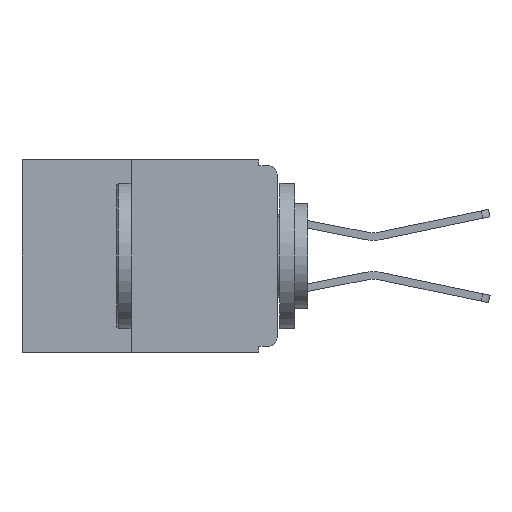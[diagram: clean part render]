
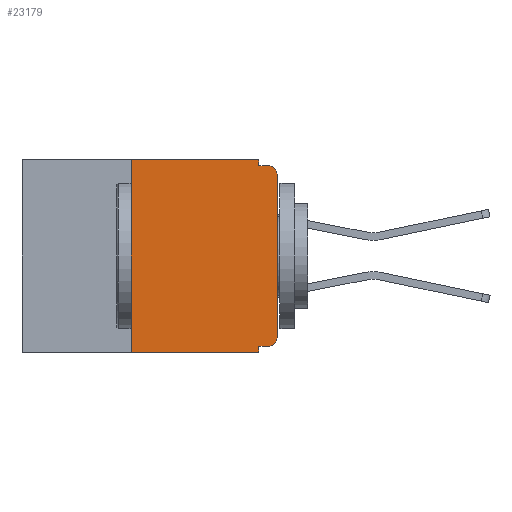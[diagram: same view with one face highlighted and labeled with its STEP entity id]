
A CAD part, left-side view. The second image highlights one B-rep face of the part: STEP entity #23179.
In plain terms, the highlighted planar face has unit normal (-1, 0, 0).
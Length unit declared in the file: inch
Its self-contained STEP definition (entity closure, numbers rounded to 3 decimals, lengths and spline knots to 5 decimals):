
#619 = AXIS2_PLACEMENT_3D ( 'NONE', #27748, #3390, #27098 ) ;
#1403 = ORIENTED_EDGE ( 'NONE', *, *, #21141, .F. ) ;
#2416 = EDGE_CURVE ( 'NONE', #32948, #7726, #2552, .T. ) ;
#2425 = EDGE_CURVE ( 'NONE', #13186, #30338, #24092, .T. ) ;
#2552 = CIRCLE ( 'NONE', #619, 0.015 ) ;
#2761 = LINE ( 'NONE', #4427, #23470 ) ;
#3285 = DIRECTION ( 'NONE',  ( -1., 0., 0. ) ) ;
#3390 = DIRECTION ( 'NONE',  ( -1., 0., 0. ) ) ;
#3770 = LINE ( 'NONE', #6785, #4599 ) ;
#3822 = VERTEX_POINT ( 'NONE', #17124 ) ;
#4195 = CARTESIAN_POINT ( 'NONE',  ( 0., 0.25, -0.33 ) ) ;
#4427 = CARTESIAN_POINT ( 'NONE',  ( 0., 0., -0.32 ) ) ;
#4599 = VECTOR ( 'NONE', #7134, 39.37008 ) ;
#4861 = DIRECTION ( 'NONE',  ( 0., 1., 0. ) ) ;
#5353 = VERTEX_POINT ( 'NONE', #21780 ) ;
#5910 = DIRECTION ( 'NONE',  ( 0., 0., 1. ) ) ;
#5989 = EDGE_CURVE ( 'NONE', #21607, #5353, #2761, .T. ) ;
#6082 = ORIENTED_EDGE ( 'NONE', *, *, #9510, .F. ) ;
#6320 = VECTOR ( 'NONE', #32234, 39.37008 ) ;
#6785 = CARTESIAN_POINT ( 'NONE',  ( 0., 0.031, 0. ) ) ;
#7110 = LINE ( 'NONE', #31302, #33940 ) ;
#7134 = DIRECTION ( 'NONE',  ( 0., 0., -1. ) ) ;
#7726 = VERTEX_POINT ( 'NONE', #27463 ) ;
#8636 = ORIENTED_EDGE ( 'NONE', *, *, #26899, .T. ) ;
#9510 = EDGE_CURVE ( 'NONE', #30338, #3822, #3770, .T. ) ;
#10314 = ORIENTED_EDGE ( 'NONE', *, *, #25846, .F. ) ;
#10710 = ORIENTED_EDGE ( 'NONE', *, *, #17851, .T. ) ;
#11234 = PLANE ( 'NONE',  #32733 ) ;
#13186 = VERTEX_POINT ( 'NONE', #15292 ) ;
#13444 = FACE_OUTER_BOUND ( 'NONE', #34259, .T. ) ;
#13531 = CARTESIAN_POINT ( 'NONE',  ( 0., 0.031, -0.33 ) ) ;
#15292 = CARTESIAN_POINT ( 'NONE',  ( 0., 0.25, 0. ) ) ;
#15488 = CARTESIAN_POINT ( 'NONE',  ( 0., 0.437, -0.33 ) ) ;
#15538 = CIRCLE ( 'NONE', #16472, 0.015 ) ;
#16472 = AXIS2_PLACEMENT_3D ( 'NONE', #19548, #3285, #22234 ) ;
#16754 = DIRECTION ( 'NONE',  ( 0., 0., -1. ) ) ;
#16958 = LINE ( 'NONE', #4195, #23244 ) ;
#17124 = CARTESIAN_POINT ( 'NONE',  ( 0., 0.031, -0.01 ) ) ;
#17563 = ORIENTED_EDGE ( 'NONE', *, *, #5989, .F. ) ;
#17851 = EDGE_CURVE ( 'NONE', #26490, #32948, #23380, .T. ) ;
#17964 = ORIENTED_EDGE ( 'NONE', *, *, #2416, .T. ) ;
#19274 = ORIENTED_EDGE ( 'NONE', *, *, #23769, .T. ) ;
#19548 = CARTESIAN_POINT ( 'NONE',  ( 0., 0.015, -0.305 ) ) ;
#20734 = LINE ( 'NONE', #13531, #6320 ) ;
#21141 = EDGE_CURVE ( 'NONE', #31419, #13186, #16958, .T. ) ;
#21607 = VERTEX_POINT ( 'NONE', #26167 ) ;
#21777 = CARTESIAN_POINT ( 'NONE',  ( 0., 0., -0.305 ) ) ;
#21780 = CARTESIAN_POINT ( 'NONE',  ( 0., 0.031, -0.32 ) ) ;
#22234 = DIRECTION ( 'NONE',  ( 0., 0., -1. ) ) ;
#22889 = CARTESIAN_POINT ( 'NONE',  ( 0., 0.25, -0.33 ) ) ;
#23179 = ADVANCED_FACE ( 'NONE', ( #13444 ), #11234, .F. ) ;
#23244 = VECTOR ( 'NONE', #28454, 39.37008 ) ;
#23262 = VECTOR ( 'NONE', #28965, 39.37008 ) ;
#23380 = LINE ( 'NONE', #27325, #29591 ) ;
#23470 = VECTOR ( 'NONE', #4861, 39.37008 ) ;
#23769 = EDGE_CURVE ( 'NONE', #21607, #26490, #15538, .T. ) ;
#24092 = LINE ( 'NONE', #29010, #23262 ) ;
#24585 = CARTESIAN_POINT ( 'NONE',  ( 0., 0.031, -0.33 ) ) ;
#25846 = EDGE_CURVE ( 'NONE', #5353, #30004, #20734, .T. ) ;
#26066 = DIRECTION ( 'NONE',  ( 0., -1., 0. ) ) ;
#26167 = CARTESIAN_POINT ( 'NONE',  ( 0., 0.015, -0.32 ) ) ;
#26490 = VERTEX_POINT ( 'NONE', #21777 ) ;
#26694 = ORIENTED_EDGE ( 'NONE', *, *, #32181, .F. ) ;
#26899 = EDGE_CURVE ( 'NONE', #31419, #30004, #28102, .T. ) ;
#27098 = DIRECTION ( 'NONE',  ( 0., 0., -1. ) ) ;
#27325 = CARTESIAN_POINT ( 'NONE',  ( 0., 0., 0. ) ) ;
#27463 = CARTESIAN_POINT ( 'NONE',  ( 0., 0.015, -0.01 ) ) ;
#27748 = CARTESIAN_POINT ( 'NONE',  ( 0., 0.015, -0.025 ) ) ;
#28102 = LINE ( 'NONE', #15488, #34333 ) ;
#28454 = DIRECTION ( 'NONE',  ( 0., 0., 1. ) ) ;
#28965 = DIRECTION ( 'NONE',  ( 0., -1., 0. ) ) ;
#29010 = CARTESIAN_POINT ( 'NONE',  ( 0., 0.437, 0. ) ) ;
#29205 = ORIENTED_EDGE ( 'NONE', *, *, #2425, .F. ) ;
#29591 = VECTOR ( 'NONE', #5910, 39.37008 ) ;
#30004 = VERTEX_POINT ( 'NONE', #24585 ) ;
#30007 = CARTESIAN_POINT ( 'NONE',  ( 0., 0.437, 0. ) ) ;
#30338 = VERTEX_POINT ( 'NONE', #31296 ) ;
#31296 = CARTESIAN_POINT ( 'NONE',  ( 0., 0.031, 0. ) ) ;
#31302 = CARTESIAN_POINT ( 'NONE',  ( 0., 0., -0.01 ) ) ;
#31356 = DIRECTION ( 'NONE',  ( 0., -1., 0. ) ) ;
#31419 = VERTEX_POINT ( 'NONE', #22889 ) ;
#32181 = EDGE_CURVE ( 'NONE', #3822, #7726, #7110, .T. ) ;
#32234 = DIRECTION ( 'NONE',  ( 0., 0., -1. ) ) ;
#32693 = DIRECTION ( 'NONE',  ( 1., 0., 0. ) ) ;
#32733 = AXIS2_PLACEMENT_3D ( 'NONE', #30007, #32693, #16754 ) ;
#32948 = VERTEX_POINT ( 'NONE', #34366 ) ;
#33940 = VECTOR ( 'NONE', #26066, 39.37008 ) ;
#34259 = EDGE_LOOP ( 'NONE', ( #10710, #17964, #26694, #6082, #29205, #1403, #8636, #10314, #17563, #19274 ) ) ;
#34333 = VECTOR ( 'NONE', #31356, 39.37008 ) ;
#34366 = CARTESIAN_POINT ( 'NONE',  ( 0., 0., -0.025 ) ) ;
